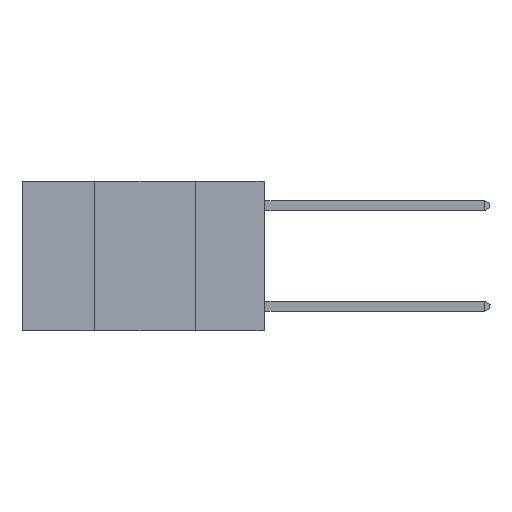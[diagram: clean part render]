
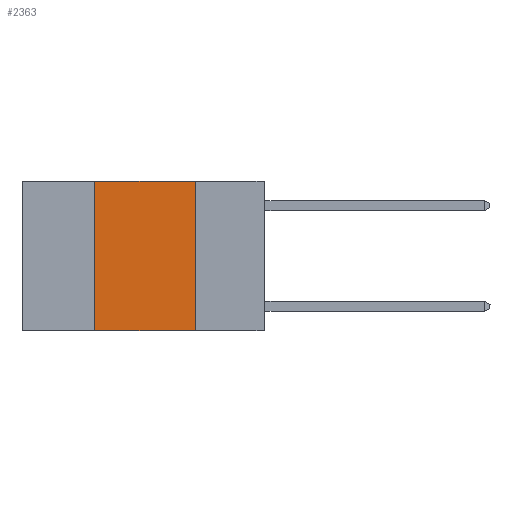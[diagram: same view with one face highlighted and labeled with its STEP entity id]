
A CAD part, left-side view. The second image highlights one B-rep face of the part: STEP entity #2363.
In plain terms, the highlighted planar face has unit normal (-1, 0, 0).
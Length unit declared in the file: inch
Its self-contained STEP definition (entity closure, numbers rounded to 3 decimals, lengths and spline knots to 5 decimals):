
#1748 = LINE ( 'NONE', #7459, #16402 ) ;
#2363 = ADVANCED_FACE ( 'NONE', ( #17048 ), #2779, .F. ) ;
#2779 = PLANE ( 'NONE',  #9685 ) ;
#3925 = CARTESIAN_POINT ( 'NONE',  ( 0., 0.17, 0. ) ) ;
#3998 = LINE ( 'NONE', #14652, #11071 ) ;
#4174 = CARTESIAN_POINT ( 'NONE',  ( 0., 0.6, -0.37 ) ) ;
#4266 = EDGE_LOOP ( 'NONE', ( #10712, #7197, #15230, #19134 ) ) ;
#4294 = DIRECTION ( 'NONE',  ( 1., 0., 0. ) ) ;
#4817 = CARTESIAN_POINT ( 'NONE',  ( 0., 0.17, 0. ) ) ;
#5417 = DIRECTION ( 'NONE',  ( 0., 0., -1. ) ) ;
#5441 = CARTESIAN_POINT ( 'NONE',  ( 0., 0.42, 0. ) ) ;
#7197 = ORIENTED_EDGE ( 'NONE', *, *, #8661, .F. ) ;
#7294 = CARTESIAN_POINT ( 'NONE',  ( 0., 0.17, -0.37 ) ) ;
#7459 = CARTESIAN_POINT ( 'NONE',  ( 0., 0.6, 0. ) ) ;
#7709 = EDGE_CURVE ( 'NONE', #13052, #7895, #9349, .T. ) ;
#7852 = EDGE_CURVE ( 'NONE', #11025, #7895, #18483, .T. ) ;
#7895 = VERTEX_POINT ( 'NONE', #7294 ) ;
#8661 = EDGE_CURVE ( 'NONE', #15726, #13052, #1748, .T. ) ;
#9349 = LINE ( 'NONE', #3925, #16871 ) ;
#9685 = AXIS2_PLACEMENT_3D ( 'NONE', #13361, #4294, #14886 ) ;
#10712 = ORIENTED_EDGE ( 'NONE', *, *, #7709, .F. ) ;
#11025 = VERTEX_POINT ( 'NONE', #11611 ) ;
#11071 = VECTOR ( 'NONE', #16156, 39.37008 ) ;
#11611 = CARTESIAN_POINT ( 'NONE',  ( 0., 0.42, -0.37 ) ) ;
#13052 = VERTEX_POINT ( 'NONE', #4817 ) ;
#13361 = CARTESIAN_POINT ( 'NONE',  ( 0., 0.6, 0. ) ) ;
#14579 = VECTOR ( 'NONE', #14765, 39.37008 ) ;
#14652 = CARTESIAN_POINT ( 'NONE',  ( 0., 0.42, 0. ) ) ;
#14765 = DIRECTION ( 'NONE',  ( 0., -1., 0. ) ) ;
#14886 = DIRECTION ( 'NONE',  ( 0., 0., -1. ) ) ;
#15230 = ORIENTED_EDGE ( 'NONE', *, *, #17606, .F. ) ;
#15726 = VERTEX_POINT ( 'NONE', #5441 ) ;
#16156 = DIRECTION ( 'NONE',  ( 0., 0., 1. ) ) ;
#16402 = VECTOR ( 'NONE', #16475, 39.37008 ) ;
#16475 = DIRECTION ( 'NONE',  ( 0., -1., 0. ) ) ;
#16871 = VECTOR ( 'NONE', #5417, 39.37008 ) ;
#17048 = FACE_OUTER_BOUND ( 'NONE', #4266, .T. ) ;
#17606 = EDGE_CURVE ( 'NONE', #11025, #15726, #3998, .T. ) ;
#18483 = LINE ( 'NONE', #4174, #14579 ) ;
#19134 = ORIENTED_EDGE ( 'NONE', *, *, #7852, .T. ) ;
